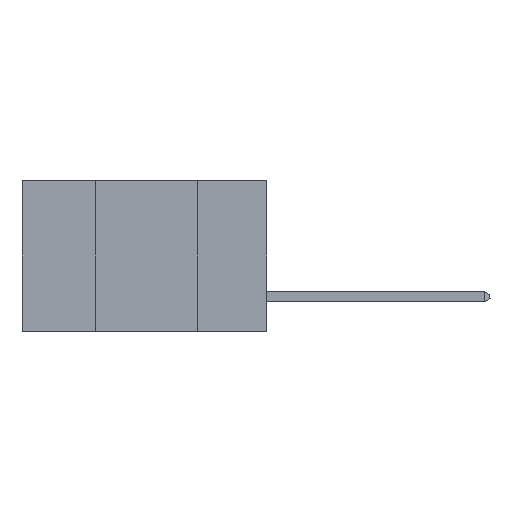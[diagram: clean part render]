
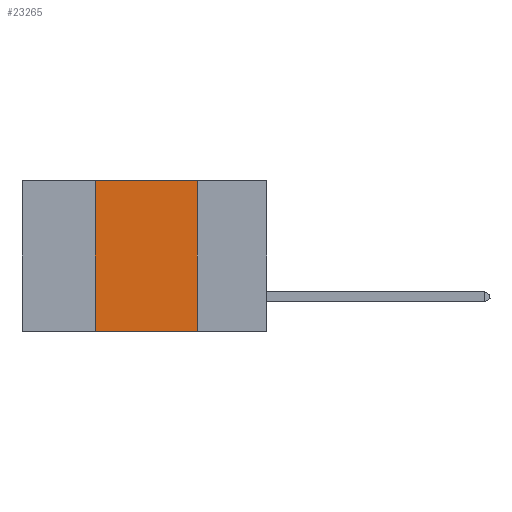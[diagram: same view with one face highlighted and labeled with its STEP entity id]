
A CAD part, left-side view. The second image highlights one B-rep face of the part: STEP entity #23265.
In plain terms, the highlighted planar face has unit normal (-1, 0, 0).
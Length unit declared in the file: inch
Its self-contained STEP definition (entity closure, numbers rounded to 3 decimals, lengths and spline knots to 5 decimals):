
#465 = DIRECTION ( 'NONE',  ( 0., -1., 0. ) ) ;
#1150 = ORIENTED_EDGE ( 'NONE', *, *, #40993, .F. ) ;
#1166 = VECTOR ( 'NONE', #21250, 39.37008 ) ;
#3226 = VERTEX_POINT ( 'NONE', #27683 ) ;
#4004 = CARTESIAN_POINT ( 'NONE',  ( 0., 0.17, -0.37 ) ) ;
#7290 = DIRECTION ( 'NONE',  ( 1., 0., 0. ) ) ;
#7305 = AXIS2_PLACEMENT_3D ( 'NONE', #23007, #7290, #8016 ) ;
#8016 = DIRECTION ( 'NONE',  ( 0., 0., -1. ) ) ;
#12349 = EDGE_CURVE ( 'NONE', #17559, #16425, #37806, .T. ) ;
#13628 = PLANE ( 'NONE',  #7305 ) ;
#15169 = LINE ( 'NONE', #29760, #16576 ) ;
#16425 = VERTEX_POINT ( 'NONE', #4004 ) ;
#16576 = VECTOR ( 'NONE', #23560, 39.37008 ) ;
#16673 = VECTOR ( 'NONE', #18475, 39.37008 ) ;
#17271 = VECTOR ( 'NONE', #465, 39.37008 ) ;
#17559 = VERTEX_POINT ( 'NONE', #18366 ) ;
#18226 = CARTESIAN_POINT ( 'NONE',  ( 0., 0.42, -0.37 ) ) ;
#18366 = CARTESIAN_POINT ( 'NONE',  ( 0., 0.17, 0. ) ) ;
#18475 = DIRECTION ( 'NONE',  ( 0., 0., 1. ) ) ;
#18486 = EDGE_CURVE ( 'NONE', #28873, #3226, #34533, .T. ) ;
#21250 = DIRECTION ( 'NONE',  ( 0., 0., -1. ) ) ;
#22214 = ORIENTED_EDGE ( 'NONE', *, *, #18486, .F. ) ;
#23007 = CARTESIAN_POINT ( 'NONE',  ( 0., 0.6, 0. ) ) ;
#23236 = LINE ( 'NONE', #32145, #17271 ) ;
#23265 = ADVANCED_FACE ( 'NONE', ( #28319 ), #13628, .F. ) ;
#23560 = DIRECTION ( 'NONE',  ( 0., -1., 0. ) ) ;
#24829 = EDGE_LOOP ( 'NONE', ( #29360, #1150, #22214, #24924 ) ) ;
#24924 = ORIENTED_EDGE ( 'NONE', *, *, #38885, .T. ) ;
#27683 = CARTESIAN_POINT ( 'NONE',  ( 0., 0.42, 0. ) ) ;
#28319 = FACE_OUTER_BOUND ( 'NONE', #24829, .T. ) ;
#28873 = VERTEX_POINT ( 'NONE', #18226 ) ;
#29360 = ORIENTED_EDGE ( 'NONE', *, *, #12349, .F. ) ;
#29760 = CARTESIAN_POINT ( 'NONE',  ( 0., 0.6, 0. ) ) ;
#32145 = CARTESIAN_POINT ( 'NONE',  ( 0., 0.6, -0.37 ) ) ;
#34533 = LINE ( 'NONE', #37274, #16673 ) ;
#37274 = CARTESIAN_POINT ( 'NONE',  ( 0., 0.42, 0. ) ) ;
#37445 = CARTESIAN_POINT ( 'NONE',  ( 0., 0.17, 0. ) ) ;
#37806 = LINE ( 'NONE', #37445, #1166 ) ;
#38885 = EDGE_CURVE ( 'NONE', #28873, #16425, #23236, .T. ) ;
#40993 = EDGE_CURVE ( 'NONE', #3226, #17559, #15169, .T. ) ;
